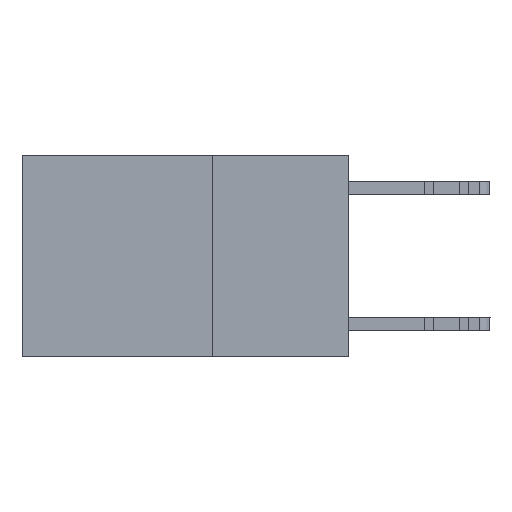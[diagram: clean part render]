
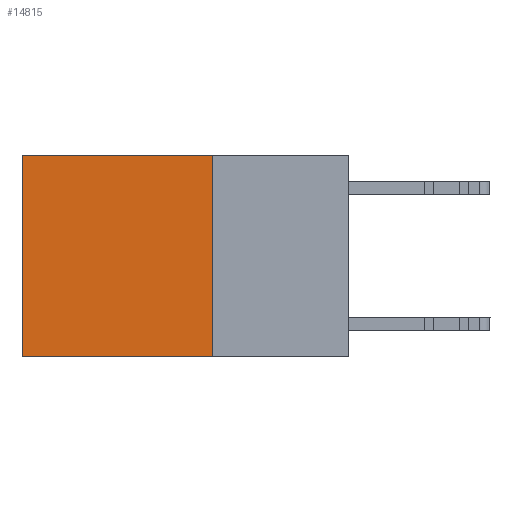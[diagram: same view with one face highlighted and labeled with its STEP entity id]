
A CAD part, left-side view. The second image highlights one B-rep face of the part: STEP entity #14815.
In plain terms, the highlighted planar face has unit normal (-1, 0, 0).
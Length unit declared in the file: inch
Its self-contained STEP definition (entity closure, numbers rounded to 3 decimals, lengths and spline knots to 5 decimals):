
#1595 = EDGE_LOOP ( 'NONE', ( #8228, #28576, #17529, #22435 ) ) ;
#2158 = EDGE_CURVE ( 'NONE', #12594, #25749, #10591, .T. ) ;
#3763 = DIRECTION ( 'NONE',  ( 0., 0., -1. ) ) ;
#3828 = DIRECTION ( 'NONE',  ( 1., 0., 0. ) ) ;
#3952 = CARTESIAN_POINT ( 'NONE',  ( 0.2625, 0.25, 0. ) ) ;
#4039 = DIRECTION ( 'NONE',  ( 0., 0., -1. ) ) ;
#4151 = PLANE ( 'NONE',  #24134 ) ;
#4340 = CARTESIAN_POINT ( 'NONE',  ( 0.2625, 0.25, 0. ) ) ;
#8228 = ORIENTED_EDGE ( 'NONE', *, *, #2158, .T. ) ;
#10110 = FACE_OUTER_BOUND ( 'NONE', #1595, .T. ) ;
#10191 = VECTOR ( 'NONE', #27460, 39.37008 ) ;
#10591 = LINE ( 'NONE', #28822, #10191 ) ;
#11328 = VECTOR ( 'NONE', #22269, 39.37008 ) ;
#12594 = VERTEX_POINT ( 'NONE', #19884 ) ;
#12694 = EDGE_CURVE ( 'NONE', #16413, #12594, #13542, .T. ) ;
#13103 = VECTOR ( 'NONE', #17113, 39.37008 ) ;
#13542 = LINE ( 'NONE', #17335, #13103 ) ;
#14251 = CARTESIAN_POINT ( 'NONE',  ( 0.2625, 0.25, 0. ) ) ;
#14815 = ADVANCED_FACE ( 'NONE', ( #10110 ), #4151, .F. ) ;
#15382 = CARTESIAN_POINT ( 'NONE',  ( 0.2625, 0.25, -0.37 ) ) ;
#15576 = EDGE_CURVE ( 'NONE', #15846, #25749, #16332, .T. ) ;
#15846 = VERTEX_POINT ( 'NONE', #15382 ) ;
#16332 = LINE ( 'NONE', #22521, #11328 ) ;
#16413 = VERTEX_POINT ( 'NONE', #14251 ) ;
#17113 = DIRECTION ( 'NONE',  ( 0., 1., 0. ) ) ;
#17335 = CARTESIAN_POINT ( 'NONE',  ( 0.2625, 0.25, 0. ) ) ;
#17529 = ORIENTED_EDGE ( 'NONE', *, *, #21709, .F. ) ;
#17566 = VECTOR ( 'NONE', #4039, 39.37008 ) ;
#17816 = LINE ( 'NONE', #4340, #17566 ) ;
#19111 = CARTESIAN_POINT ( 'NONE',  ( 0.2625, 0.6, -0.37 ) ) ;
#19884 = CARTESIAN_POINT ( 'NONE',  ( 0.2625, 0.6, 0. ) ) ;
#21709 = EDGE_CURVE ( 'NONE', #16413, #15846, #17816, .T. ) ;
#22269 = DIRECTION ( 'NONE',  ( 0., 1., 0. ) ) ;
#22435 = ORIENTED_EDGE ( 'NONE', *, *, #12694, .T. ) ;
#22521 = CARTESIAN_POINT ( 'NONE',  ( 0.2625, 0.25, -0.37 ) ) ;
#24134 = AXIS2_PLACEMENT_3D ( 'NONE', #3952, #3828, #3763 ) ;
#25749 = VERTEX_POINT ( 'NONE', #19111 ) ;
#27460 = DIRECTION ( 'NONE',  ( 0., 0., -1. ) ) ;
#28576 = ORIENTED_EDGE ( 'NONE', *, *, #15576, .F. ) ;
#28822 = CARTESIAN_POINT ( 'NONE',  ( 0.2625, 0.6, 0. ) ) ;
